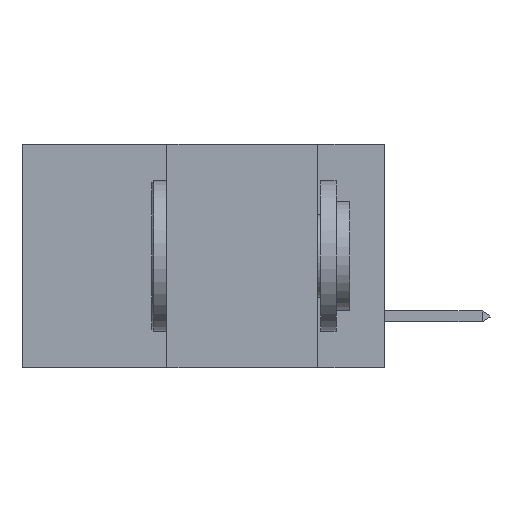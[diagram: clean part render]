
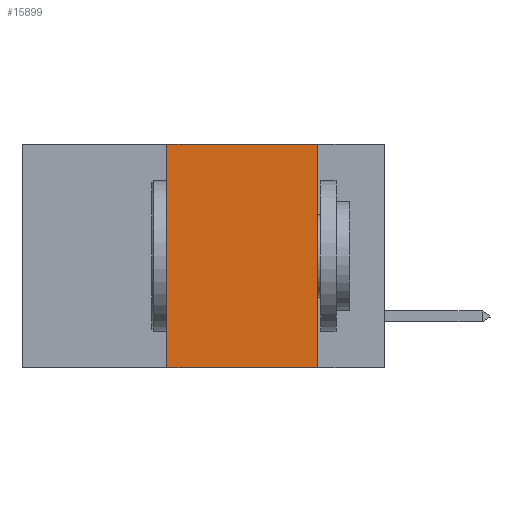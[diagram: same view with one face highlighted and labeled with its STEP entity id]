
A CAD part, left-side view. The second image highlights one B-rep face of the part: STEP entity #15899.
In plain terms, the highlighted planar face has unit normal (-1, 0, 0).
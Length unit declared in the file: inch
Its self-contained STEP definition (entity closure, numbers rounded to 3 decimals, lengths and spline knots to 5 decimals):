
#216 = EDGE_CURVE ( 'NONE', #1784, #22300, #8615, .T. ) ;
#1784 = VERTEX_POINT ( 'NONE', #12762 ) ;
#2978 = VERTEX_POINT ( 'NONE', #10664 ) ;
#3344 = VECTOR ( 'NONE', #21864, 39.37008 ) ;
#3402 = VECTOR ( 'NONE', #21443, 39.37008 ) ;
#3650 = CARTESIAN_POINT ( 'NONE',  ( 0., 0.6, 0. ) ) ;
#4710 = CARTESIAN_POINT ( 'NONE',  ( 0., 0.6, 0. ) ) ;
#5218 = VECTOR ( 'NONE', #6913, 39.37008 ) ;
#5367 = EDGE_CURVE ( 'NONE', #14060, #1784, #16672, .T. ) ;
#5436 = DIRECTION ( 'NONE',  ( 1., 0., 0. ) ) ;
#5600 = ORIENTED_EDGE ( 'NONE', *, *, #8780, .F. ) ;
#5861 = CARTESIAN_POINT ( 'NONE',  ( 0., 0.11, 0. ) ) ;
#6913 = DIRECTION ( 'NONE',  ( 0., -1., 0. ) ) ;
#8094 = CARTESIAN_POINT ( 'NONE',  ( 0., 0.11, 0. ) ) ;
#8105 = LINE ( 'NONE', #5861, #3402 ) ;
#8272 = ORIENTED_EDGE ( 'NONE', *, *, #10949, .T. ) ;
#8602 = FACE_OUTER_BOUND ( 'NONE', #18754, .T. ) ;
#8615 = LINE ( 'NONE', #4710, #3344 ) ;
#8780 = EDGE_CURVE ( 'NONE', #22300, #2978, #8105, .T. ) ;
#9062 = ORIENTED_EDGE ( 'NONE', *, *, #5367, .F. ) ;
#9892 = LINE ( 'NONE', #15544, #5218 ) ;
#10657 = PLANE ( 'NONE',  #11675 ) ;
#10664 = CARTESIAN_POINT ( 'NONE',  ( 0., 0.11, -0.37 ) ) ;
#10878 = ORIENTED_EDGE ( 'NONE', *, *, #216, .F. ) ;
#10949 = EDGE_CURVE ( 'NONE', #14060, #2978, #9892, .T. ) ;
#11675 = AXIS2_PLACEMENT_3D ( 'NONE', #3650, #5436, #17579 ) ;
#12762 = CARTESIAN_POINT ( 'NONE',  ( 0., 0.36, 0. ) ) ;
#14024 = CARTESIAN_POINT ( 'NONE',  ( 0., 0.36, -0.37 ) ) ;
#14060 = VERTEX_POINT ( 'NONE', #14024 ) ;
#15122 = CARTESIAN_POINT ( 'NONE',  ( 0., 0.36, 0. ) ) ;
#15544 = CARTESIAN_POINT ( 'NONE',  ( 0., 0.6, -0.37 ) ) ;
#15584 = VECTOR ( 'NONE', #16853, 39.37008 ) ;
#15899 = ADVANCED_FACE ( 'NONE', ( #8602 ), #10657, .F. ) ;
#16672 = LINE ( 'NONE', #15122, #15584 ) ;
#16853 = DIRECTION ( 'NONE',  ( 0., 0., 1. ) ) ;
#17579 = DIRECTION ( 'NONE',  ( 0., 0., -1. ) ) ;
#18754 = EDGE_LOOP ( 'NONE', ( #5600, #10878, #9062, #8272 ) ) ;
#21443 = DIRECTION ( 'NONE',  ( 0., 0., -1. ) ) ;
#21864 = DIRECTION ( 'NONE',  ( 0., -1., 0. ) ) ;
#22300 = VERTEX_POINT ( 'NONE', #8094 ) ;
